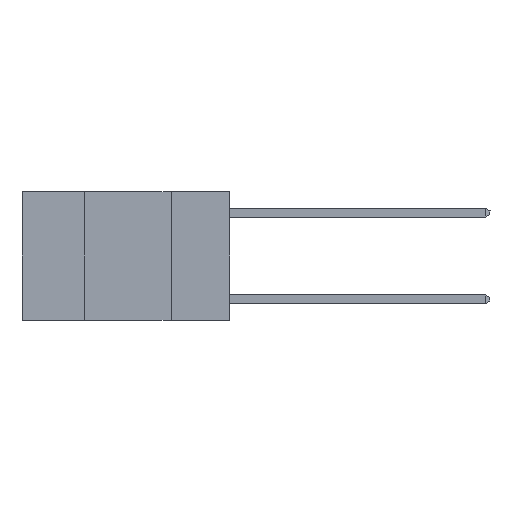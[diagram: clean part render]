
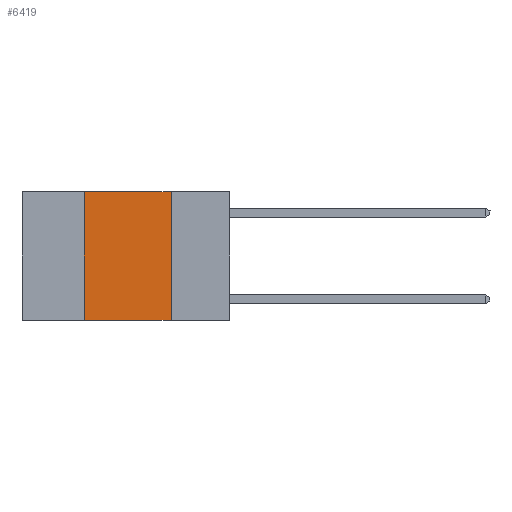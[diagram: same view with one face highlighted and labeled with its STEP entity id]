
A CAD part, left-side view. The second image highlights one B-rep face of the part: STEP entity #6419.
In plain terms, the highlighted planar face has unit normal (-1, 0, 0).
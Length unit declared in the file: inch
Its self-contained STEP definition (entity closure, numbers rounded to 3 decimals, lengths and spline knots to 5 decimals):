
#936 = FACE_OUTER_BOUND ( 'NONE', #5331, .T. ) ;
#1041 = DIRECTION ( 'NONE',  ( 0., 0., -1. ) ) ;
#1412 = AXIS2_PLACEMENT_3D ( 'NONE', #8373, #3318, #9224 ) ;
#1911 = VERTEX_POINT ( 'NONE', #7066 ) ;
#2032 = VECTOR ( 'NONE', #3926, 39.37008 ) ;
#2243 = CARTESIAN_POINT ( 'NONE',  ( 0., 0.17, 0. ) ) ;
#2348 = LINE ( 'NONE', #2735, #10594 ) ;
#2432 = PLANE ( 'NONE',  #1412 ) ;
#2564 = VERTEX_POINT ( 'NONE', #6775 ) ;
#2685 = EDGE_CURVE ( 'NONE', #2564, #5210, #8550, .T. ) ;
#2735 = CARTESIAN_POINT ( 'NONE',  ( 0., 0.17, 0. ) ) ;
#3318 = DIRECTION ( 'NONE',  ( 1., 0., 0. ) ) ;
#3728 = VECTOR ( 'NONE', #8289, 39.37008 ) ;
#3926 = DIRECTION ( 'NONE',  ( 0., 0., 1. ) ) ;
#3962 = CARTESIAN_POINT ( 'NONE',  ( 0., 0.42, 0. ) ) ;
#4213 = VERTEX_POINT ( 'NONE', #2243 ) ;
#4909 = CARTESIAN_POINT ( 'NONE',  ( 0., 0.6, 0. ) ) ;
#5210 = VERTEX_POINT ( 'NONE', #8577 ) ;
#5236 = CARTESIAN_POINT ( 'NONE',  ( 0., 0.6, -0.37 ) ) ;
#5331 = EDGE_LOOP ( 'NONE', ( #7286, #7251, #7156, #7136 ) ) ;
#6064 = LINE ( 'NONE', #5236, #8254 ) ;
#6419 = ADVANCED_FACE ( 'NONE', ( #936 ), #2432, .F. ) ;
#6775 = CARTESIAN_POINT ( 'NONE',  ( 0., 0.42, -0.37 ) ) ;
#7025 = EDGE_CURVE ( 'NONE', #2564, #1911, #6064, .T. ) ;
#7066 = CARTESIAN_POINT ( 'NONE',  ( 0., 0.17, -0.37 ) ) ;
#7136 = ORIENTED_EDGE ( 'NONE', *, *, #7025, .T. ) ;
#7156 = ORIENTED_EDGE ( 'NONE', *, *, #2685, .F. ) ;
#7251 = ORIENTED_EDGE ( 'NONE', *, *, #7413, .F. ) ;
#7286 = ORIENTED_EDGE ( 'NONE', *, *, #8878, .F. ) ;
#7413 = EDGE_CURVE ( 'NONE', #5210, #4213, #10498, .T. ) ;
#8254 = VECTOR ( 'NONE', #9433, 39.37008 ) ;
#8289 = DIRECTION ( 'NONE',  ( 0., -1., 0. ) ) ;
#8373 = CARTESIAN_POINT ( 'NONE',  ( 0., 0.6, 0. ) ) ;
#8550 = LINE ( 'NONE', #3962, #2032 ) ;
#8577 = CARTESIAN_POINT ( 'NONE',  ( 0., 0.42, 0. ) ) ;
#8878 = EDGE_CURVE ( 'NONE', #4213, #1911, #2348, .T. ) ;
#9224 = DIRECTION ( 'NONE',  ( 0., 0., -1. ) ) ;
#9433 = DIRECTION ( 'NONE',  ( 0., -1., 0. ) ) ;
#10498 = LINE ( 'NONE', #4909, #3728 ) ;
#10594 = VECTOR ( 'NONE', #1041, 39.37008 ) ;
